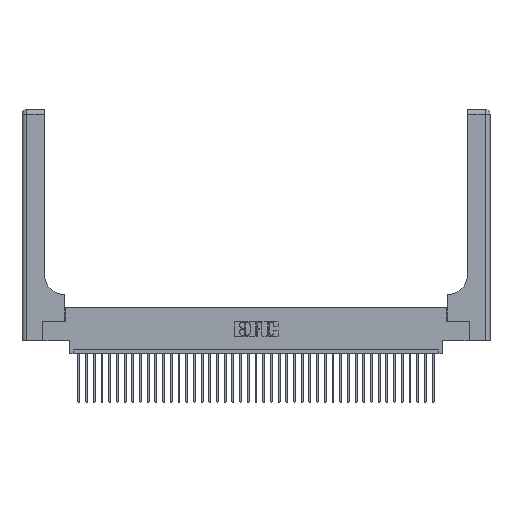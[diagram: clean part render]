
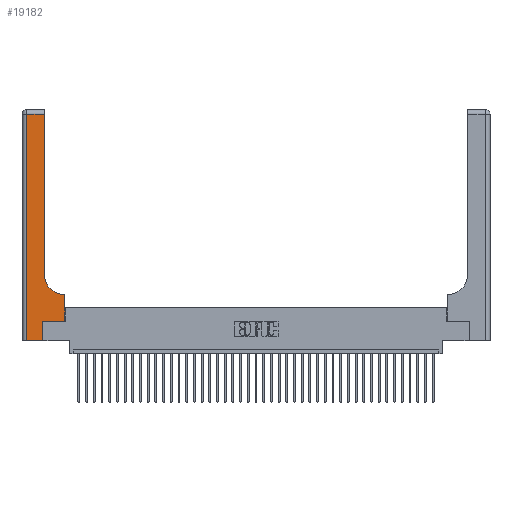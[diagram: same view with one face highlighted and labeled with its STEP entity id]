
A CAD part, top view. The second image highlights one B-rep face of the part: STEP entity #19182.
In plain terms, the highlighted planar face has unit normal (0, 0, 1).
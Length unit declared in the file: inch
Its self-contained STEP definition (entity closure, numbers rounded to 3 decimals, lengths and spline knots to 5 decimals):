
#70 = CARTESIAN_POINT ( 'NONE',  ( 0.5585, 0.25, 0.37 ) ) ;
#277 = ORIENTED_EDGE ( 'NONE', *, *, #31059, .T. ) ;
#383 = CARTESIAN_POINT ( 'NONE',  ( 0.5415, 0.85, 0.37 ) ) ;
#461 = VERTEX_POINT ( 'NONE', #30567 ) ;
#556 = VECTOR ( 'NONE', #27189, 39.37008 ) ;
#1538 = CARTESIAN_POINT ( 'NONE',  ( 0.2915, 0.6, 0.37 ) ) ;
#2352 = EDGE_CURVE ( 'NONE', #12887, #13987, #20830, .T. ) ;
#2549 = VECTOR ( 'NONE', #10685, 39.37008 ) ;
#2631 = CARTESIAN_POINT ( 'NONE',  ( 0.269, 0.25, 0.37 ) ) ;
#2921 = ORIENTED_EDGE ( 'NONE', *, *, #33637, .T. ) ;
#3398 = CARTESIAN_POINT ( 'NONE',  ( 0., 3., 0.37 ) ) ;
#3951 = CARTESIAN_POINT ( 'NONE',  ( 0.06, 0., 0.37 ) ) ;
#4132 = DIRECTION ( 'NONE',  ( 1., 0., 0. ) ) ;
#4483 = LINE ( 'NONE', #26694, #11597 ) ;
#5526 = CARTESIAN_POINT ( 'NONE',  ( 0.2915, 3., 0.37 ) ) ;
#5888 = DIRECTION ( 'NONE',  ( 1., 0., 0. ) ) ;
#6323 = ORIENTED_EDGE ( 'NONE', *, *, #2352, .T. ) ;
#7272 = FACE_OUTER_BOUND ( 'NONE', #16217, .T. ) ;
#7541 = VERTEX_POINT ( 'NONE', #25809 ) ;
#7585 = EDGE_CURVE ( 'NONE', #38384, #29838, #22339, .T. ) ;
#7595 = CARTESIAN_POINT ( 'NONE',  ( 0.5585, 0.25, 0.37 ) ) ;
#9071 = VERTEX_POINT ( 'NONE', #32013 ) ;
#10147 = AXIS2_PLACEMENT_3D ( 'NONE', #383, #38038, #4132 ) ;
#10685 = DIRECTION ( 'NONE',  ( 0., 1., 0. ) ) ;
#11597 = VECTOR ( 'NONE', #26996, 39.37008 ) ;
#11902 = CARTESIAN_POINT ( 'NONE',  ( 0.2915, 0.85, 0.37 ) ) ;
#12887 = VERTEX_POINT ( 'NONE', #11902 ) ;
#13126 = ORIENTED_EDGE ( 'NONE', *, *, #27116, .T. ) ;
#13150 = DIRECTION ( 'NONE',  ( 1., 0., 0. ) ) ;
#13987 = VERTEX_POINT ( 'NONE', #31188 ) ;
#15071 = VECTOR ( 'NONE', #5888, 39.37008 ) ;
#16217 = EDGE_LOOP ( 'NONE', ( #6323, #2921, #277, #30589, #26569, #35977, #36470, #25746, #13126 ) ) ;
#16225 = EDGE_CURVE ( 'NONE', #34005, #7541, #19372, .T. ) ;
#16232 = VERTEX_POINT ( 'NONE', #2631 ) ;
#16748 = AXIS2_PLACEMENT_3D ( 'NONE', #3398, #21512, #27926 ) ;
#18060 = DIRECTION ( 'NONE',  ( -1., 0., 0. ) ) ;
#18997 = LINE ( 'NONE', #26831, #33502 ) ;
#19182 = ADVANCED_FACE ( 'NONE', ( #7272 ), #37324, .F. ) ;
#19372 = LINE ( 'NONE', #21275, #15071 ) ;
#20830 = LINE ( 'NONE', #5526, #556 ) ;
#21275 = CARTESIAN_POINT ( 'NONE',  ( 0., 0., 0.37 ) ) ;
#21324 = CARTESIAN_POINT ( 'NONE',  ( 0.269, 0.25, 0.37 ) ) ;
#21512 = DIRECTION ( 'NONE',  ( 0., 0., -1. ) ) ;
#22325 = VECTOR ( 'NONE', #29448, 39.37008 ) ;
#22339 = LINE ( 'NONE', #7595, #2549 ) ;
#22762 = DIRECTION ( 'NONE',  ( 0., 1., 0. ) ) ;
#25746 = ORIENTED_EDGE ( 'NONE', *, *, #32905, .T. ) ;
#25809 = CARTESIAN_POINT ( 'NONE',  ( 0.269, 0., 0.37 ) ) ;
#26560 = CARTESIAN_POINT ( 'NONE',  ( 0.5585, 0.6, 0.37 ) ) ;
#26569 = ORIENTED_EDGE ( 'NONE', *, *, #29111, .T. ) ;
#26694 = CARTESIAN_POINT ( 'NONE',  ( 0.06, 3., 0.37 ) ) ;
#26831 = CARTESIAN_POINT ( 'NONE',  ( 0., 2.94, 0.37 ) ) ;
#26996 = DIRECTION ( 'NONE',  ( 0., -1., 0. ) ) ;
#27116 = EDGE_CURVE ( 'NONE', #9071, #12887, #31723, .T. ) ;
#27189 = DIRECTION ( 'NONE',  ( 0., 1., 0. ) ) ;
#27926 = DIRECTION ( 'NONE',  ( -1., 0., 0. ) ) ;
#28675 = LINE ( 'NONE', #1538, #22325 ) ;
#29111 = EDGE_CURVE ( 'NONE', #7541, #16232, #30682, .T. ) ;
#29448 = DIRECTION ( 'NONE',  ( -1., 0., 0. ) ) ;
#29838 = VERTEX_POINT ( 'NONE', #26560 ) ;
#29865 = VECTOR ( 'NONE', #13150, 39.37008 ) ;
#30567 = CARTESIAN_POINT ( 'NONE',  ( 0.06, 2.94, 0.37 ) ) ;
#30589 = ORIENTED_EDGE ( 'NONE', *, *, #16225, .T. ) ;
#30682 = LINE ( 'NONE', #35628, #37874 ) ;
#31059 = EDGE_CURVE ( 'NONE', #461, #34005, #4483, .T. ) ;
#31188 = CARTESIAN_POINT ( 'NONE',  ( 0.2915, 2.94, 0.37 ) ) ;
#31723 = CIRCLE ( 'NONE', #10147, 0.25 ) ;
#32013 = CARTESIAN_POINT ( 'NONE',  ( 0.5415, 0.6, 0.37 ) ) ;
#32905 = EDGE_CURVE ( 'NONE', #29838, #9071, #28675, .T. ) ;
#33502 = VECTOR ( 'NONE', #18060, 39.37008 ) ;
#33637 = EDGE_CURVE ( 'NONE', #13987, #461, #18997, .T. ) ;
#34005 = VERTEX_POINT ( 'NONE', #3951 ) ;
#35628 = CARTESIAN_POINT ( 'NONE',  ( 0.269, 0., 0.37 ) ) ;
#35977 = ORIENTED_EDGE ( 'NONE', *, *, #36535, .T. ) ;
#36470 = ORIENTED_EDGE ( 'NONE', *, *, #7585, .T. ) ;
#36535 = EDGE_CURVE ( 'NONE', #16232, #38384, #39992, .T. ) ;
#37324 = PLANE ( 'NONE',  #16748 ) ;
#37874 = VECTOR ( 'NONE', #22762, 39.37008 ) ;
#38038 = DIRECTION ( 'NONE',  ( 0., 0., -1. ) ) ;
#38384 = VERTEX_POINT ( 'NONE', #70 ) ;
#39992 = LINE ( 'NONE', #21324, #29865 ) ;
